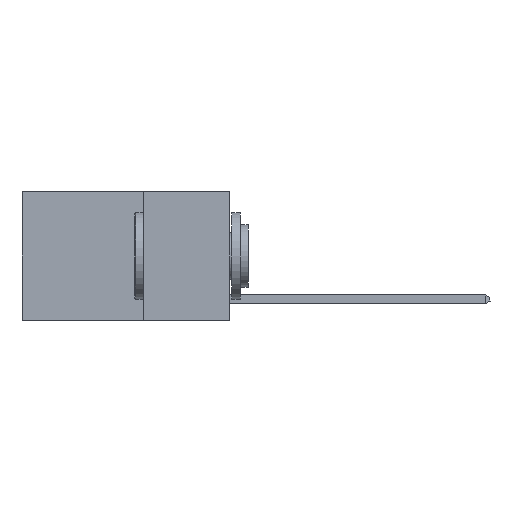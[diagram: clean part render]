
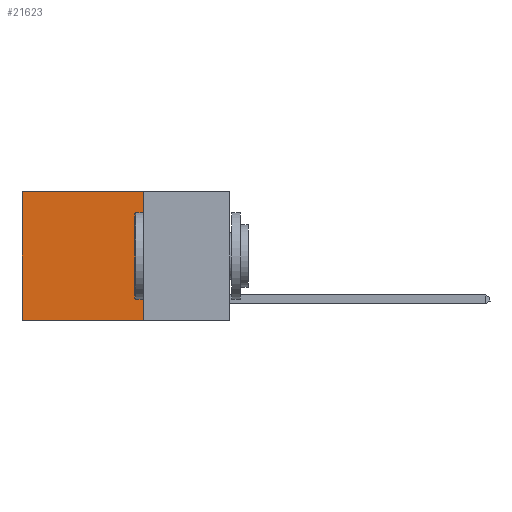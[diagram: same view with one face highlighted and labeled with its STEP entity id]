
A CAD part, left-side view. The second image highlights one B-rep face of the part: STEP entity #21623.
In plain terms, the highlighted planar face has unit normal (-1, 0, 0).
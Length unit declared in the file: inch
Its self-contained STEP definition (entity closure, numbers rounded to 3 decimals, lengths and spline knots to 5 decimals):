
#833 = LINE ( 'NONE', #8994, #20782 ) ;
#1049 = DIRECTION ( 'NONE',  ( 0., 0., -1. ) ) ;
#1694 = ORIENTED_EDGE ( 'NONE', *, *, #3645, .T. ) ;
#1893 = VERTEX_POINT ( 'NONE', #24500 ) ;
#3522 = LINE ( 'NONE', #19513, #9416 ) ;
#3532 = DIRECTION ( 'NONE',  ( 1., 0., 0. ) ) ;
#3595 = ORIENTED_EDGE ( 'NONE', *, *, #6922, .F. ) ;
#3645 = EDGE_CURVE ( 'NONE', #1893, #17140, #833, .T. ) ;
#4058 = CARTESIAN_POINT ( 'NONE',  ( 0.2625, 0.6, -0.37 ) ) ;
#4857 = CARTESIAN_POINT ( 'NONE',  ( 0.2625, 0.25, -0.37 ) ) ;
#5648 = DIRECTION ( 'NONE',  ( 0., 0., -1. ) ) ;
#6357 = EDGE_CURVE ( 'NONE', #16972, #13461, #3522, .T. ) ;
#6696 = DIRECTION ( 'NONE',  ( 0., 1., 0. ) ) ;
#6922 = EDGE_CURVE ( 'NONE', #13461, #17140, #15586, .T. ) ;
#8994 = CARTESIAN_POINT ( 'NONE',  ( 0.2625, 0.6, 0. ) ) ;
#9416 = VECTOR ( 'NONE', #5648, 39.37008 ) ;
#9474 = ORIENTED_EDGE ( 'NONE', *, *, #14616, .T. ) ;
#13251 = PLANE ( 'NONE',  #20032 ) ;
#13461 = VERTEX_POINT ( 'NONE', #4857 ) ;
#14616 = EDGE_CURVE ( 'NONE', #16972, #1893, #16416, .T. ) ;
#15418 = CARTESIAN_POINT ( 'NONE',  ( 0.2625, 0.25, 0. ) ) ;
#15586 = LINE ( 'NONE', #21137, #25501 ) ;
#16416 = LINE ( 'NONE', #24522, #21078 ) ;
#16972 = VERTEX_POINT ( 'NONE', #21077 ) ;
#17140 = VERTEX_POINT ( 'NONE', #4058 ) ;
#17424 = DIRECTION ( 'NONE',  ( 0., 0., -1. ) ) ;
#17958 = EDGE_LOOP ( 'NONE', ( #1694, #3595, #20784, #9474 ) ) ;
#18993 = FACE_OUTER_BOUND ( 'NONE', #17958, .T. ) ;
#19513 = CARTESIAN_POINT ( 'NONE',  ( 0.2625, 0.25, 0. ) ) ;
#20032 = AXIS2_PLACEMENT_3D ( 'NONE', #15418, #3532, #17424 ) ;
#20782 = VECTOR ( 'NONE', #1049, 39.37008 ) ;
#20784 = ORIENTED_EDGE ( 'NONE', *, *, #6357, .F. ) ;
#21077 = CARTESIAN_POINT ( 'NONE',  ( 0.2625, 0.25, 0. ) ) ;
#21078 = VECTOR ( 'NONE', #6696, 39.37008 ) ;
#21137 = CARTESIAN_POINT ( 'NONE',  ( 0.2625, 0.25, -0.37 ) ) ;
#21623 = ADVANCED_FACE ( 'NONE', ( #18993 ), #13251, .F. ) ;
#23104 = DIRECTION ( 'NONE',  ( 0., 1., 0. ) ) ;
#24500 = CARTESIAN_POINT ( 'NONE',  ( 0.2625, 0.6, 0. ) ) ;
#24522 = CARTESIAN_POINT ( 'NONE',  ( 0.2625, 0.25, 0. ) ) ;
#25501 = VECTOR ( 'NONE', #23104, 39.37008 ) ;
